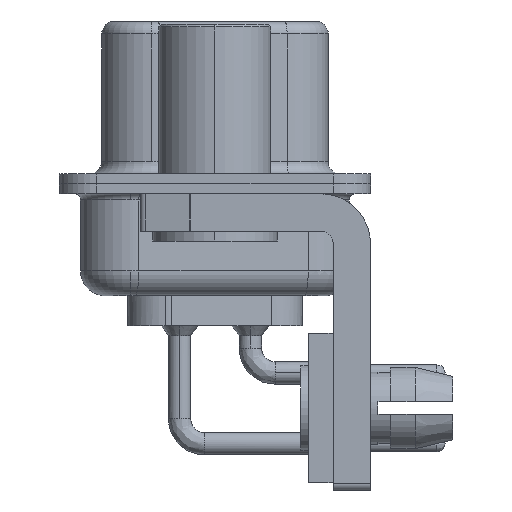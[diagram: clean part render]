
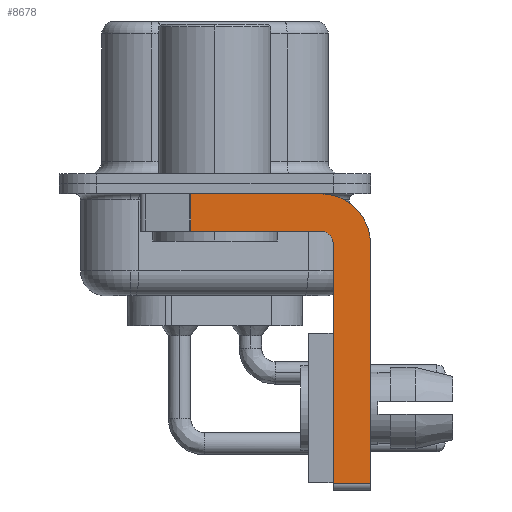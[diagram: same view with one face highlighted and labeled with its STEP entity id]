
A CAD part, left-side view. The second image highlights one B-rep face of the part: STEP entity #8678.
In plain terms, the highlighted planar face has unit normal (-1, 0, 0).
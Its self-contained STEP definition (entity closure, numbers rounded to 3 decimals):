
#1009 = VECTOR ( 'NONE', #7746, 1000. ) ;
#1283 = EDGE_CURVE ( 'NONE', #5161, #30261, #2733, .T. ) ;
#1375 = CARTESIAN_POINT ( 'NONE',  ( -2.9, 0.978, -1.9 ) ) ;
#1442 = DIRECTION ( 'NONE',  ( 1., 0., 0. ) ) ;
#1629 = CARTESIAN_POINT ( 'NONE',  ( -2.9, -4.25, -0.4 ) ) ;
#2733 = LINE ( 'NONE', #17650, #8447 ) ;
#2921 = FACE_OUTER_BOUND ( 'NONE', #13098, .T. ) ;
#2958 = ORIENTED_EDGE ( 'NONE', *, *, #26676, .F. ) ;
#3478 = ORIENTED_EDGE ( 'NONE', *, *, #5992, .F. ) ;
#3898 = CARTESIAN_POINT ( 'NONE',  ( -2.9, 0.978, -0.4 ) ) ;
#5082 = DIRECTION ( 'NONE',  ( -1., 0., 0. ) ) ;
#5161 = VERTEX_POINT ( 'NONE', #5233 ) ;
#5180 = CARTESIAN_POINT ( 'NONE',  ( -2.9, 0.978, -1.9 ) ) ;
#5233 = CARTESIAN_POINT ( 'NONE',  ( -2.9, -6.25, -2.4 ) ) ;
#5939 = VECTOR ( 'NONE', #10106, 1000. ) ;
#5992 = EDGE_CURVE ( 'NONE', #7450, #5161, #28642, .T. ) ;
#6704 = LINE ( 'NONE', #5180, #5939 ) ;
#6866 = CARTESIAN_POINT ( 'NONE',  ( -2.9, -4.25, -1.9 ) ) ;
#7390 = VERTEX_POINT ( 'NONE', #3898 ) ;
#7450 = VERTEX_POINT ( 'NONE', #1629 ) ;
#7746 = DIRECTION ( 'NONE',  ( 0., -1., 0. ) ) ;
#7950 = CARTESIAN_POINT ( 'NONE',  ( -2.9, -4.75, -12.05 ) ) ;
#8101 = AXIS2_PLACEMENT_3D ( 'NONE', #16164, #1442, #18625 ) ;
#8222 = EDGE_CURVE ( 'NONE', #7390, #7450, #25823, .T. ) ;
#8447 = VECTOR ( 'NONE', #15526, 1000. ) ;
#8548 = DIRECTION ( 'NONE',  ( 0., 0., 1. ) ) ;
#8678 = ADVANCED_FACE ( 'NONE', ( #2921 ), #30732, .F. ) ;
#9415 = CARTESIAN_POINT ( 'NONE',  ( -2.9, 3., -0.4 ) ) ;
#10106 = DIRECTION ( 'NONE',  ( 0., 0., -1. ) ) ;
#10772 = ORIENTED_EDGE ( 'NONE', *, *, #8222, .F. ) ;
#10991 = CARTESIAN_POINT ( 'NONE',  ( -2.9, -4.25, -1.9 ) ) ;
#11490 = CARTESIAN_POINT ( 'NONE',  ( -2.9, -4.75, -2.4 ) ) ;
#12793 = ORIENTED_EDGE ( 'NONE', *, *, #23953, .T. ) ;
#13098 = EDGE_LOOP ( 'NONE', ( #10772, #12793, #2958, #30771, #26944, #20737, #23289, #3478 ) ) ;
#13137 = CARTESIAN_POINT ( 'NONE',  ( -2.9, -4.25, -2.4 ) ) ;
#13717 = VECTOR ( 'NONE', #24032, 1000. ) ;
#13892 = VERTEX_POINT ( 'NONE', #6866 ) ;
#14130 = LINE ( 'NONE', #22356, #1009 ) ;
#14189 = LINE ( 'NONE', #10991, #20604 ) ;
#14979 = VERTEX_POINT ( 'NONE', #11490 ) ;
#15526 = DIRECTION ( 'NONE',  ( 0., 0., -1. ) ) ;
#15594 = DIRECTION ( 'NONE',  ( 0., 0., -1. ) ) ;
#15902 = EDGE_CURVE ( 'NONE', #14979, #13892, #16399, .T. ) ;
#15962 = EDGE_CURVE ( 'NONE', #29829, #30261, #14130, .T. ) ;
#16035 = VECTOR ( 'NONE', #8548, 1000. ) ;
#16164 = CARTESIAN_POINT ( 'NONE',  ( -2.9, -4.25, -2.4 ) ) ;
#16399 = CIRCLE ( 'NONE', #16538, 0.5 ) ;
#16538 = AXIS2_PLACEMENT_3D ( 'NONE', #19750, #5082, #22152 ) ;
#17650 = CARTESIAN_POINT ( 'NONE',  ( -2.9, -6.25, -2.4 ) ) ;
#18448 = CARTESIAN_POINT ( 'NONE',  ( -2.9, -4.75, -12.3 ) ) ;
#18453 = VERTEX_POINT ( 'NONE', #1375 ) ;
#18625 = DIRECTION ( 'NONE',  ( 0., 0., -1. ) ) ;
#19201 = CARTESIAN_POINT ( 'NONE',  ( -2.9, -6.25, -12.05 ) ) ;
#19248 = AXIS2_PLACEMENT_3D ( 'NONE', #13137, #30135, #15594 ) ;
#19750 = CARTESIAN_POINT ( 'NONE',  ( -2.9, -4.25, -2.4 ) ) ;
#20604 = VECTOR ( 'NONE', #25538, 1000. ) ;
#20737 = ORIENTED_EDGE ( 'NONE', *, *, #15962, .T. ) ;
#22152 = DIRECTION ( 'NONE',  ( 0., 0., 1. ) ) ;
#22356 = CARTESIAN_POINT ( 'NONE',  ( -2.9, -4.25, -12.05 ) ) ;
#22445 = LINE ( 'NONE', #18448, #16035 ) ;
#23289 = ORIENTED_EDGE ( 'NONE', *, *, #1283, .F. ) ;
#23953 = EDGE_CURVE ( 'NONE', #7390, #18453, #6704, .T. ) ;
#24032 = DIRECTION ( 'NONE',  ( 0., -1., 0. ) ) ;
#25538 = DIRECTION ( 'NONE',  ( 0., 1., 0. ) ) ;
#25823 = LINE ( 'NONE', #9415, #13717 ) ;
#26676 = EDGE_CURVE ( 'NONE', #13892, #18453, #14189, .T. ) ;
#26944 = ORIENTED_EDGE ( 'NONE', *, *, #27207, .F. ) ;
#27207 = EDGE_CURVE ( 'NONE', #29829, #14979, #22445, .T. ) ;
#28642 = CIRCLE ( 'NONE', #19248, 2. ) ;
#29829 = VERTEX_POINT ( 'NONE', #7950 ) ;
#30135 = DIRECTION ( 'NONE',  ( 1., 0., 0. ) ) ;
#30261 = VERTEX_POINT ( 'NONE', #19201 ) ;
#30732 = PLANE ( 'NONE',  #8101 ) ;
#30771 = ORIENTED_EDGE ( 'NONE', *, *, #15902, .F. ) ;
